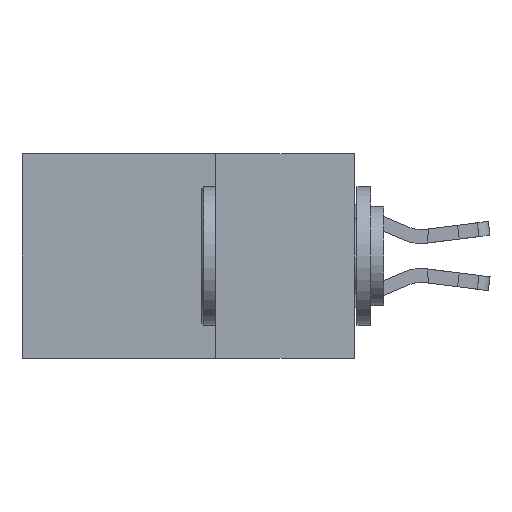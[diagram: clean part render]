
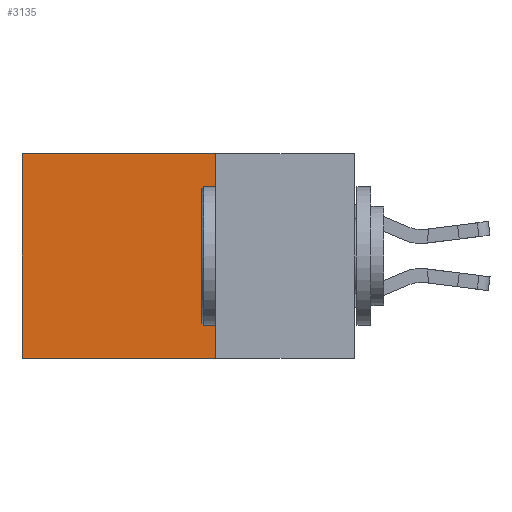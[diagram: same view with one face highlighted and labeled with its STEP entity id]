
A CAD part, left-side view. The second image highlights one B-rep face of the part: STEP entity #3135.
In plain terms, the highlighted planar face has unit normal (-1, 0, 0).
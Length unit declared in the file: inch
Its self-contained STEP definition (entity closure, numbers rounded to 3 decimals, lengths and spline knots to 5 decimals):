
#281 = AXIS2_PLACEMENT_3D ( 'NONE', #9738, #5760, #7629 ) ;
#315 = VERTEX_POINT ( 'NONE', #4105 ) ;
#340 = CARTESIAN_POINT ( 'NONE',  ( 0.298, 0.25, -0.37 ) ) ;
#1312 = CARTESIAN_POINT ( 'NONE',  ( 0.298, 0.6, 0. ) ) ;
#1419 = DIRECTION ( 'NONE',  ( 0., 0., -1. ) ) ;
#1671 = ORIENTED_EDGE ( 'NONE', *, *, #8966, .F. ) ;
#2625 = CARTESIAN_POINT ( 'NONE',  ( 0.298, 0.25, -0.37 ) ) ;
#3135 = ADVANCED_FACE ( 'NONE', ( #6764 ), #5639, .F. ) ;
#3216 = VERTEX_POINT ( 'NONE', #8629 ) ;
#3735 = VERTEX_POINT ( 'NONE', #340 ) ;
#3908 = ORIENTED_EDGE ( 'NONE', *, *, #4341, .F. ) ;
#4105 = CARTESIAN_POINT ( 'NONE',  ( 0.298, 0.25, 0. ) ) ;
#4341 = EDGE_CURVE ( 'NONE', #3735, #6417, #10689, .T. ) ;
#4981 = ORIENTED_EDGE ( 'NONE', *, *, #6410, .T. ) ;
#5639 = PLANE ( 'NONE',  #281 ) ;
#5760 = DIRECTION ( 'NONE',  ( 1., 0., 0. ) ) ;
#6250 = CARTESIAN_POINT ( 'NONE',  ( 0.298, 0.25, 0. ) ) ;
#6410 = EDGE_CURVE ( 'NONE', #3216, #6417, #11090, .T. ) ;
#6417 = VERTEX_POINT ( 'NONE', #6672 ) ;
#6672 = CARTESIAN_POINT ( 'NONE',  ( 0.298, 0.6, -0.37 ) ) ;
#6764 = FACE_OUTER_BOUND ( 'NONE', #10381, .T. ) ;
#7543 = VECTOR ( 'NONE', #10490, 39.37008 ) ;
#7629 = DIRECTION ( 'NONE',  ( 0., 0., -1. ) ) ;
#7631 = CARTESIAN_POINT ( 'NONE',  ( 0.298, 0.25, 0. ) ) ;
#7985 = VECTOR ( 'NONE', #11769, 39.37008 ) ;
#8629 = CARTESIAN_POINT ( 'NONE',  ( 0.298, 0.6, 0. ) ) ;
#8966 = EDGE_CURVE ( 'NONE', #315, #3735, #9732, .T. ) ;
#9188 = LINE ( 'NONE', #7631, #7543 ) ;
#9732 = LINE ( 'NONE', #6250, #11605 ) ;
#9738 = CARTESIAN_POINT ( 'NONE',  ( 0.298, 0.25, 0. ) ) ;
#10002 = DIRECTION ( 'NONE',  ( 0., 1., 0. ) ) ;
#10109 = VECTOR ( 'NONE', #10002, 39.37008 ) ;
#10381 = EDGE_LOOP ( 'NONE', ( #4981, #3908, #1671, #12112 ) ) ;
#10490 = DIRECTION ( 'NONE',  ( 0., 1., 0. ) ) ;
#10689 = LINE ( 'NONE', #2625, #10109 ) ;
#11090 = LINE ( 'NONE', #1312, #7985 ) ;
#11291 = EDGE_CURVE ( 'NONE', #315, #3216, #9188, .T. ) ;
#11605 = VECTOR ( 'NONE', #1419, 39.37008 ) ;
#11769 = DIRECTION ( 'NONE',  ( 0., 0., -1. ) ) ;
#12112 = ORIENTED_EDGE ( 'NONE', *, *, #11291, .T. ) ;
